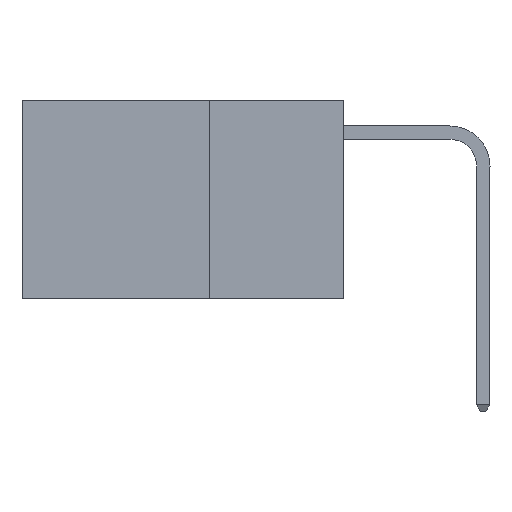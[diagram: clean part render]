
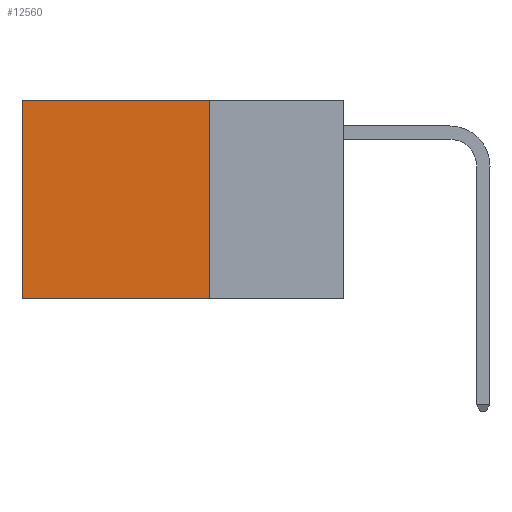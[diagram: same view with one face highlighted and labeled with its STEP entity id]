
A CAD part, left-side view. The second image highlights one B-rep face of the part: STEP entity #12560.
In plain terms, the highlighted planar face has unit normal (-1, 0, 0).
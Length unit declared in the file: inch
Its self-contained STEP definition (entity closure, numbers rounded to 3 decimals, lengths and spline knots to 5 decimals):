
#143 = EDGE_CURVE ( 'NONE', #15783, #19894, #12322, .T. ) ;
#1265 = DIRECTION ( 'NONE',  ( 0., 0., -1. ) ) ;
#1882 = EDGE_CURVE ( 'NONE', #13160, #12412, #22711, .T. ) ;
#2946 = LINE ( 'NONE', #19442, #22768 ) ;
#3452 = CARTESIAN_POINT ( 'NONE',  ( 0.2625, 0.6, -0.37 ) ) ;
#3475 = ORIENTED_EDGE ( 'NONE', *, *, #1882, .F. ) ;
#3885 = ORIENTED_EDGE ( 'NONE', *, *, #8667, .F. ) ;
#4591 = ORIENTED_EDGE ( 'NONE', *, *, #23041, .T. ) ;
#6522 = CARTESIAN_POINT ( 'NONE',  ( 0.2625, 0.25, -0.37 ) ) ;
#6577 = CARTESIAN_POINT ( 'NONE',  ( 0.2625, 0.25, 0. ) ) ;
#6823 = CARTESIAN_POINT ( 'NONE',  ( 0.2625, 0.25, 0. ) ) ;
#7212 = VECTOR ( 'NONE', #13842, 39.37008 ) ;
#8062 = CARTESIAN_POINT ( 'NONE',  ( 0.2625, 0.6, 0. ) ) ;
#8667 = EDGE_CURVE ( 'NONE', #12412, #19894, #2946, .T. ) ;
#9449 = DIRECTION ( 'NONE',  ( 0., 0., -1. ) ) ;
#10902 = PLANE ( 'NONE',  #22869 ) ;
#11799 = DIRECTION ( 'NONE',  ( 0., 1., 0. ) ) ;
#12322 = LINE ( 'NONE', #8062, #7212 ) ;
#12412 = VERTEX_POINT ( 'NONE', #6522 ) ;
#12560 = ADVANCED_FACE ( 'NONE', ( #14497 ), #10902, .F. ) ;
#12803 = DIRECTION ( 'NONE',  ( 1., 0., 0. ) ) ;
#13101 = VECTOR ( 'NONE', #9449, 39.37008 ) ;
#13160 = VERTEX_POINT ( 'NONE', #6823 ) ;
#13842 = DIRECTION ( 'NONE',  ( 0., 0., -1. ) ) ;
#14302 = DIRECTION ( 'NONE',  ( 0., 1., 0. ) ) ;
#14497 = FACE_OUTER_BOUND ( 'NONE', #21058, .T. ) ;
#15783 = VERTEX_POINT ( 'NONE', #18849 ) ;
#16188 = VECTOR ( 'NONE', #14302, 39.37008 ) ;
#18849 = CARTESIAN_POINT ( 'NONE',  ( 0.2625, 0.6, 0. ) ) ;
#19442 = CARTESIAN_POINT ( 'NONE',  ( 0.2625, 0.25, -0.37 ) ) ;
#19894 = VERTEX_POINT ( 'NONE', #3452 ) ;
#20919 = CARTESIAN_POINT ( 'NONE',  ( 0.2625, 0.25, 0. ) ) ;
#21058 = EDGE_LOOP ( 'NONE', ( #21673, #3885, #3475, #4591 ) ) ;
#21673 = ORIENTED_EDGE ( 'NONE', *, *, #143, .T. ) ;
#21893 = LINE ( 'NONE', #6577, #16188 ) ;
#22711 = LINE ( 'NONE', #20919, #13101 ) ;
#22768 = VECTOR ( 'NONE', #11799, 39.37008 ) ;
#22869 = AXIS2_PLACEMENT_3D ( 'NONE', #24301, #12803, #1265 ) ;
#23041 = EDGE_CURVE ( 'NONE', #13160, #15783, #21893, .T. ) ;
#24301 = CARTESIAN_POINT ( 'NONE',  ( 0.2625, 0.25, 0. ) ) ;
